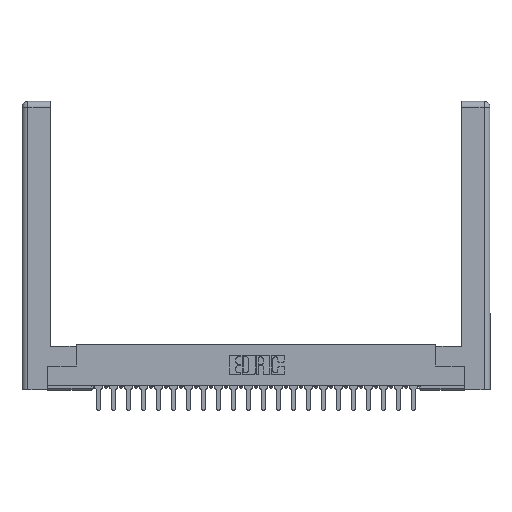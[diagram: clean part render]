
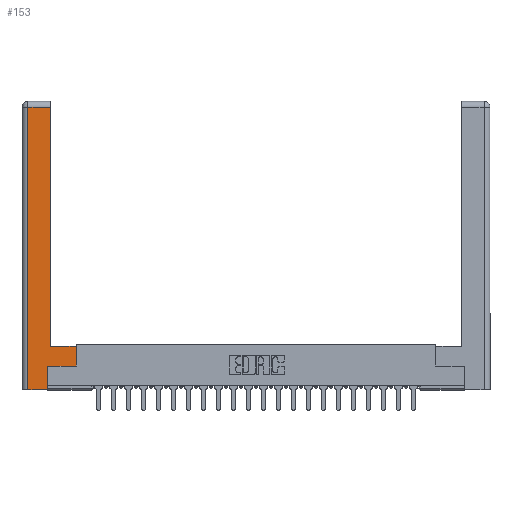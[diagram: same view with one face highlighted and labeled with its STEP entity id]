
A CAD part, top view. The second image highlights one B-rep face of the part: STEP entity #153.
In plain terms, the highlighted planar face has unit normal (0, 0, 1).
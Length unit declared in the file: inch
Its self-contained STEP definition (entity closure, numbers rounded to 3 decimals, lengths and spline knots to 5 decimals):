
#145 = DIRECTION ( 'NONE',  ( 0., 1., 0. ) ) ;
#153 = ADVANCED_FACE ( 'NONE', ( #7001 ), #7006, .F. ) ;
#243 = VECTOR ( 'NONE', #16222, 39.37008 ) ;
#461 = CARTESIAN_POINT ( 'NONE',  ( 0.295, 2.94, 0. ) ) ;
#1045 = VECTOR ( 'NONE', #2801, 39.37008 ) ;
#1206 = CARTESIAN_POINT ( 'NONE',  ( 0.265, 0., 0. ) ) ;
#1333 = DIRECTION ( 'NONE',  ( -1., 0., 0. ) ) ;
#1638 = CARTESIAN_POINT ( 'NONE',  ( 0.295, 3., 0. ) ) ;
#2040 = VECTOR ( 'NONE', #8000, 39.37008 ) ;
#2313 = ORIENTED_EDGE ( 'NONE', *, *, #19719, .T. ) ;
#2485 = VECTOR ( 'NONE', #16831, 39.37008 ) ;
#2606 = CARTESIAN_POINT ( 'NONE',  ( 0.0615, 0., 0. ) ) ;
#2801 = DIRECTION ( 'NONE',  ( -1., 0., 0. ) ) ;
#2979 = DIRECTION ( 'NONE',  ( 0., 0., -1. ) ) ;
#3710 = CARTESIAN_POINT ( 'NONE',  ( 0.565, 0.245, 0. ) ) ;
#3797 = VERTEX_POINT ( 'NONE', #3710 ) ;
#4020 = EDGE_CURVE ( 'NONE', #3797, #15626, #24438, .T. ) ;
#4384 = VERTEX_POINT ( 'NONE', #9114 ) ;
#4443 = AXIS2_PLACEMENT_3D ( 'NONE', #14455, #2979, #1333 ) ;
#4694 = CARTESIAN_POINT ( 'NONE',  ( 0.565, 0.245, 0. ) ) ;
#5832 = CARTESIAN_POINT ( 'NONE',  ( 0.265, 0., 0. ) ) ;
#7001 = FACE_OUTER_BOUND ( 'NONE', #14271, .T. ) ;
#7006 = PLANE ( 'NONE',  #4443 ) ;
#7213 = CARTESIAN_POINT ( 'NONE',  ( 0.0615, 2.94, 0. ) ) ;
#7505 = VECTOR ( 'NONE', #17102, 39.37008 ) ;
#7572 = LINE ( 'NONE', #1638, #2485 ) ;
#7590 = ORIENTED_EDGE ( 'NONE', *, *, #15706, .T. ) ;
#7695 = LINE ( 'NONE', #17006, #16855 ) ;
#8000 = DIRECTION ( 'NONE',  ( 0., -1., 0. ) ) ;
#8166 = CARTESIAN_POINT ( 'NONE',  ( 0.565, 0.45, 0. ) ) ;
#8394 = DIRECTION ( 'NONE',  ( 0., 1., 0. ) ) ;
#8398 = VECTOR ( 'NONE', #8394, 39.37008 ) ;
#8927 = EDGE_CURVE ( 'NONE', #4384, #9163, #7572, .T. ) ;
#9114 = CARTESIAN_POINT ( 'NONE',  ( 0.295, 0.45, 0. ) ) ;
#9157 = ORIENTED_EDGE ( 'NONE', *, *, #8927, .T. ) ;
#9163 = VERTEX_POINT ( 'NONE', #461 ) ;
#10251 = EDGE_CURVE ( 'NONE', #19416, #13326, #20838, .T. ) ;
#11298 = ORIENTED_EDGE ( 'NONE', *, *, #11829, .T. ) ;
#11669 = VECTOR ( 'NONE', #14615, 39.37008 ) ;
#11764 = LINE ( 'NONE', #12380, #1045 ) ;
#11829 = EDGE_CURVE ( 'NONE', #23299, #3797, #15409, .T. ) ;
#12380 = CARTESIAN_POINT ( 'NONE',  ( 0.295, 0.45, 0. ) ) ;
#12815 = EDGE_CURVE ( 'NONE', #13326, #23299, #7695, .T. ) ;
#12960 = CARTESIAN_POINT ( 'NONE',  ( 0.0615, 2.94, 0. ) ) ;
#13326 = VERTEX_POINT ( 'NONE', #1206 ) ;
#13835 = EDGE_CURVE ( 'NONE', #15626, #4384, #11764, .T. ) ;
#14271 = EDGE_LOOP ( 'NONE', ( #9157, #2313, #7590, #17201, #22711, #11298, #19601, #22370 ) ) ;
#14455 = CARTESIAN_POINT ( 'NONE',  ( 0., 0., 0. ) ) ;
#14615 = DIRECTION ( 'NONE',  ( -1., 0., 0. ) ) ;
#15409 = LINE ( 'NONE', #4694, #243 ) ;
#15626 = VERTEX_POINT ( 'NONE', #8166 ) ;
#15706 = EDGE_CURVE ( 'NONE', #19518, #19416, #20766, .T. ) ;
#16222 = DIRECTION ( 'NONE',  ( 1., 0., 0. ) ) ;
#16687 = LINE ( 'NONE', #12960, #11669 ) ;
#16831 = DIRECTION ( 'NONE',  ( 0., 1., 0. ) ) ;
#16855 = VECTOR ( 'NONE', #145, 39.37008 ) ;
#17006 = CARTESIAN_POINT ( 'NONE',  ( 0.265, 0.245, 0. ) ) ;
#17102 = DIRECTION ( 'NONE',  ( 1., 0., 0. ) ) ;
#17201 = ORIENTED_EDGE ( 'NONE', *, *, #10251, .T. ) ;
#17907 = CARTESIAN_POINT ( 'NONE',  ( 0.565, 0.45, 0. ) ) ;
#19365 = CARTESIAN_POINT ( 'NONE',  ( 0.0615, 0., 0. ) ) ;
#19416 = VERTEX_POINT ( 'NONE', #2606 ) ;
#19518 = VERTEX_POINT ( 'NONE', #7213 ) ;
#19601 = ORIENTED_EDGE ( 'NONE', *, *, #4020, .T. ) ;
#19719 = EDGE_CURVE ( 'NONE', #9163, #19518, #16687, .T. ) ;
#20766 = LINE ( 'NONE', #19365, #2040 ) ;
#20838 = LINE ( 'NONE', #5832, #7505 ) ;
#22370 = ORIENTED_EDGE ( 'NONE', *, *, #13835, .T. ) ;
#22711 = ORIENTED_EDGE ( 'NONE', *, *, #12815, .T. ) ;
#23299 = VERTEX_POINT ( 'NONE', #24012 ) ;
#24012 = CARTESIAN_POINT ( 'NONE',  ( 0.265, 0.245, 0. ) ) ;
#24438 = LINE ( 'NONE', #17907, #8398 ) ;
